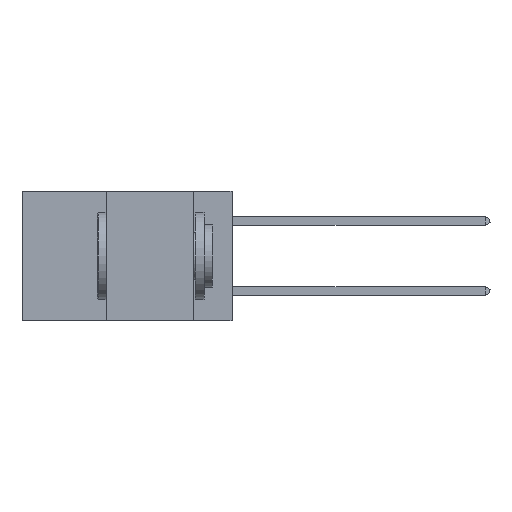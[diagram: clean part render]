
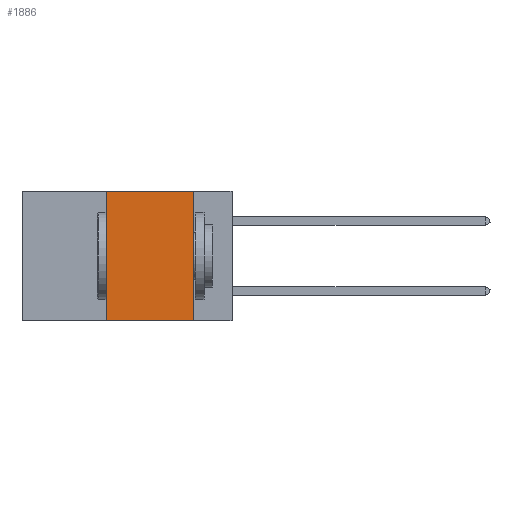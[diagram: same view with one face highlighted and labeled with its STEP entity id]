
A CAD part, left-side view. The second image highlights one B-rep face of the part: STEP entity #1886.
In plain terms, the highlighted planar face has unit normal (-1, 0, 0).
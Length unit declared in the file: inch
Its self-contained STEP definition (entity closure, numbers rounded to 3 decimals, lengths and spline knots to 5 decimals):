
#251 = CARTESIAN_POINT ( 'NONE',  ( 0., 0.11, -0.37 ) ) ;
#796 = VECTOR ( 'NONE', #5109, 39.37008 ) ;
#1886 = ADVANCED_FACE ( 'NONE', ( #10960 ), #11946, .F. ) ;
#1964 = CARTESIAN_POINT ( 'NONE',  ( 0., 0.6, 0. ) ) ;
#2011 = DIRECTION ( 'NONE',  ( 0., 0., -1. ) ) ;
#2343 = VECTOR ( 'NONE', #19778, 39.37008 ) ;
#3721 = DIRECTION ( 'NONE',  ( 0., 0., -1. ) ) ;
#3761 = DIRECTION ( 'NONE',  ( 1., 0., 0. ) ) ;
#3928 = DIRECTION ( 'NONE',  ( 0., -1., 0. ) ) ;
#3966 = AXIS2_PLACEMENT_3D ( 'NONE', #5385, #3761, #3721 ) ;
#5109 = DIRECTION ( 'NONE',  ( 0., -1., 0. ) ) ;
#5372 = LINE ( 'NONE', #18282, #796 ) ;
#5385 = CARTESIAN_POINT ( 'NONE',  ( 0., 0.6, 0. ) ) ;
#6429 = LINE ( 'NONE', #1964, #21361 ) ;
#7947 = ORIENTED_EDGE ( 'NONE', *, *, #23857, .F. ) ;
#8200 = EDGE_CURVE ( 'NONE', #8986, #19484, #5372, .T. ) ;
#8616 = CARTESIAN_POINT ( 'NONE',  ( 0., 0.36, 0. ) ) ;
#8791 = VERTEX_POINT ( 'NONE', #18335 ) ;
#8986 = VERTEX_POINT ( 'NONE', #15159 ) ;
#9719 = LINE ( 'NONE', #17110, #23385 ) ;
#10466 = EDGE_CURVE ( 'NONE', #18373, #19484, #9719, .T. ) ;
#10960 = FACE_OUTER_BOUND ( 'NONE', #19083, .T. ) ;
#11946 = PLANE ( 'NONE',  #3966 ) ;
#12377 = ORIENTED_EDGE ( 'NONE', *, *, #10466, .F. ) ;
#12955 = ORIENTED_EDGE ( 'NONE', *, *, #20867, .F. ) ;
#14130 = ORIENTED_EDGE ( 'NONE', *, *, #8200, .T. ) ;
#15159 = CARTESIAN_POINT ( 'NONE',  ( 0., 0.36, -0.37 ) ) ;
#17110 = CARTESIAN_POINT ( 'NONE',  ( 0., 0.11, 0. ) ) ;
#18282 = CARTESIAN_POINT ( 'NONE',  ( 0., 0.6, -0.37 ) ) ;
#18335 = CARTESIAN_POINT ( 'NONE',  ( 0., 0.36, 0. ) ) ;
#18373 = VERTEX_POINT ( 'NONE', #22751 ) ;
#19083 = EDGE_LOOP ( 'NONE', ( #12377, #7947, #12955, #14130 ) ) ;
#19484 = VERTEX_POINT ( 'NONE', #251 ) ;
#19778 = DIRECTION ( 'NONE',  ( 0., 0., 1. ) ) ;
#20867 = EDGE_CURVE ( 'NONE', #8986, #8791, #22920, .T. ) ;
#21361 = VECTOR ( 'NONE', #3928, 39.37008 ) ;
#22751 = CARTESIAN_POINT ( 'NONE',  ( 0., 0.11, 0. ) ) ;
#22920 = LINE ( 'NONE', #8616, #2343 ) ;
#23385 = VECTOR ( 'NONE', #2011, 39.37008 ) ;
#23857 = EDGE_CURVE ( 'NONE', #8791, #18373, #6429, .T. ) ;
